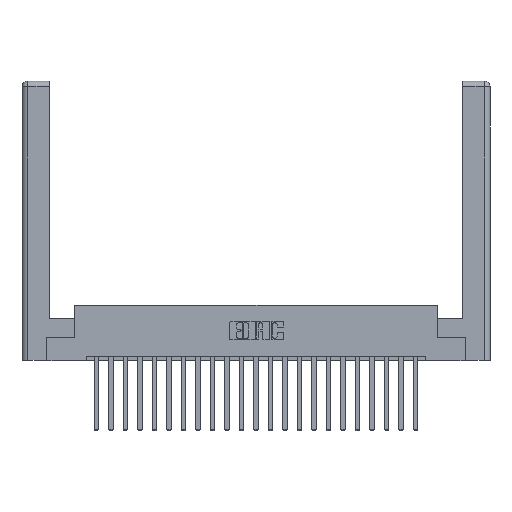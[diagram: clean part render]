
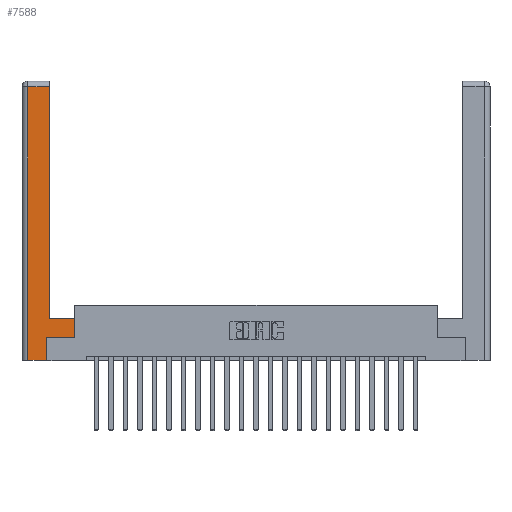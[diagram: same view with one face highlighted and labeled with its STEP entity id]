
A CAD part, top view. The second image highlights one B-rep face of the part: STEP entity #7588.
In plain terms, the highlighted planar face has unit normal (0, 0, 1).
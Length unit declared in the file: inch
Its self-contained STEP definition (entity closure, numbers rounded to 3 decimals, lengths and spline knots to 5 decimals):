
#217 = VERTEX_POINT ( 'NONE', #1875 ) ;
#823 = VECTOR ( 'NONE', #3533, 39.37008 ) ;
#1358 = EDGE_CURVE ( 'NONE', #16073, #2686, #17697, .T. ) ;
#1541 = VECTOR ( 'NONE', #6503, 39.37008 ) ;
#1634 = CARTESIAN_POINT ( 'NONE',  ( 0.565, 0.245, 0. ) ) ;
#1803 = DIRECTION ( 'NONE',  ( -1., 0., 0. ) ) ;
#1842 = CARTESIAN_POINT ( 'NONE',  ( 0.565, 0.45, 0. ) ) ;
#1875 = CARTESIAN_POINT ( 'NONE',  ( 0.295, 0.45, 0. ) ) ;
#2211 = DIRECTION ( 'NONE',  ( -1., 0., 0. ) ) ;
#2686 = VERTEX_POINT ( 'NONE', #17726 ) ;
#2884 = VECTOR ( 'NONE', #2211, 39.37008 ) ;
#2906 = ORIENTED_EDGE ( 'NONE', *, *, #17331, .T. ) ;
#3533 = DIRECTION ( 'NONE',  ( 1., 0., 0. ) ) ;
#3650 = CARTESIAN_POINT ( 'NONE',  ( 0.0615, 0., 0. ) ) ;
#4027 = VERTEX_POINT ( 'NONE', #8881 ) ;
#4689 = EDGE_CURVE ( 'NONE', #2686, #6115, #20026, .T. ) ;
#5917 = LINE ( 'NONE', #21075, #17660 ) ;
#6115 = VERTEX_POINT ( 'NONE', #1634 ) ;
#6325 = VECTOR ( 'NONE', #14421, 39.37008 ) ;
#6503 = DIRECTION ( 'NONE',  ( 1., 0., 0. ) ) ;
#7284 = ORIENTED_EDGE ( 'NONE', *, *, #18682, .T. ) ;
#7588 = ADVANCED_FACE ( 'NONE', ( #22588 ), #11265, .F. ) ;
#8224 = VECTOR ( 'NONE', #11640, 39.37008 ) ;
#8226 = LINE ( 'NONE', #3650, #6325 ) ;
#8881 = CARTESIAN_POINT ( 'NONE',  ( 0.295, 2.94, 0. ) ) ;
#8962 = VERTEX_POINT ( 'NONE', #20269 ) ;
#9207 = LINE ( 'NONE', #14492, #2884 ) ;
#9683 = CARTESIAN_POINT ( 'NONE',  ( 0.565, 0.45, 0. ) ) ;
#11265 = PLANE ( 'NONE',  #12274 ) ;
#11640 = DIRECTION ( 'NONE',  ( 0., 1., 0. ) ) ;
#11670 = ORIENTED_EDGE ( 'NONE', *, *, #20769, .T. ) ;
#11767 = VERTEX_POINT ( 'NONE', #9683 ) ;
#12198 = LINE ( 'NONE', #1842, #18089 ) ;
#12274 = AXIS2_PLACEMENT_3D ( 'NONE', #18350, #16820, #21822 ) ;
#12515 = ORIENTED_EDGE ( 'NONE', *, *, #1358, .T. ) ;
#13025 = CARTESIAN_POINT ( 'NONE',  ( 0.0615, 0., 0. ) ) ;
#13386 = ORIENTED_EDGE ( 'NONE', *, *, #14525, .T. ) ;
#13534 = CARTESIAN_POINT ( 'NONE',  ( 0.265, 0.245, 0. ) ) ;
#13567 = VERTEX_POINT ( 'NONE', #13025 ) ;
#13885 = CARTESIAN_POINT ( 'NONE',  ( 0.565, 0.245, 0. ) ) ;
#14257 = EDGE_LOOP ( 'NONE', ( #20064, #7284, #14442, #2906, #12515, #14724, #13386, #11670 ) ) ;
#14421 = DIRECTION ( 'NONE',  ( 0., -1., 0. ) ) ;
#14442 = ORIENTED_EDGE ( 'NONE', *, *, #16572, .T. ) ;
#14492 = CARTESIAN_POINT ( 'NONE',  ( 0.295, 0.45, 0. ) ) ;
#14525 = EDGE_CURVE ( 'NONE', #6115, #11767, #12198, .T. ) ;
#14724 = ORIENTED_EDGE ( 'NONE', *, *, #4689, .T. ) ;
#15906 = DIRECTION ( 'NONE',  ( 0., 1., 0. ) ) ;
#16016 = CARTESIAN_POINT ( 'NONE',  ( 0.265, 0., 0. ) ) ;
#16073 = VERTEX_POINT ( 'NONE', #17612 ) ;
#16296 = LINE ( 'NONE', #16016, #823 ) ;
#16572 = EDGE_CURVE ( 'NONE', #8962, #13567, #8226, .T. ) ;
#16820 = DIRECTION ( 'NONE',  ( 0., 0., -1. ) ) ;
#17331 = EDGE_CURVE ( 'NONE', #13567, #16073, #16296, .T. ) ;
#17612 = CARTESIAN_POINT ( 'NONE',  ( 0.265, 0., 0. ) ) ;
#17660 = VECTOR ( 'NONE', #1803, 39.37008 ) ;
#17697 = LINE ( 'NONE', #13534, #8224 ) ;
#17726 = CARTESIAN_POINT ( 'NONE',  ( 0.265, 0.245, 0. ) ) ;
#17752 = DIRECTION ( 'NONE',  ( 0., 1., 0. ) ) ;
#18089 = VECTOR ( 'NONE', #15906, 39.37008 ) ;
#18350 = CARTESIAN_POINT ( 'NONE',  ( 0., 0., 0. ) ) ;
#18413 = VECTOR ( 'NONE', #17752, 39.37008 ) ;
#18682 = EDGE_CURVE ( 'NONE', #4027, #8962, #5917, .T. ) ;
#18946 = LINE ( 'NONE', #22594, #18413 ) ;
#20026 = LINE ( 'NONE', #13885, #1541 ) ;
#20064 = ORIENTED_EDGE ( 'NONE', *, *, #20616, .T. ) ;
#20269 = CARTESIAN_POINT ( 'NONE',  ( 0.0615, 2.94, 0. ) ) ;
#20616 = EDGE_CURVE ( 'NONE', #217, #4027, #18946, .T. ) ;
#20769 = EDGE_CURVE ( 'NONE', #11767, #217, #9207, .T. ) ;
#21075 = CARTESIAN_POINT ( 'NONE',  ( 0.0615, 2.94, 0. ) ) ;
#21822 = DIRECTION ( 'NONE',  ( -1., 0., 0. ) ) ;
#22588 = FACE_OUTER_BOUND ( 'NONE', #14257, .T. ) ;
#22594 = CARTESIAN_POINT ( 'NONE',  ( 0.295, 3., 0. ) ) ;
